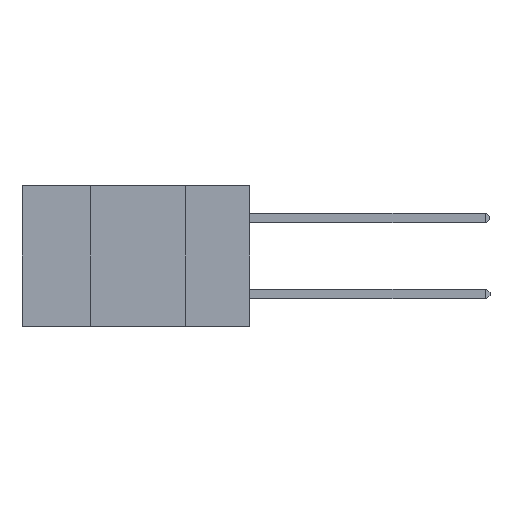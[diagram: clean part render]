
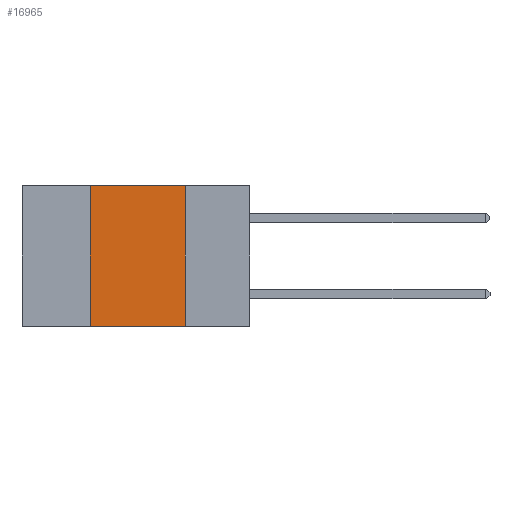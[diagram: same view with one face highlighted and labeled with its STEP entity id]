
A CAD part, left-side view. The second image highlights one B-rep face of the part: STEP entity #16965.
In plain terms, the highlighted planar face has unit normal (-1, 0, 0).
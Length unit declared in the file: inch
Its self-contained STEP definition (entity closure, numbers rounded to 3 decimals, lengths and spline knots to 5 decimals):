
#75 = VERTEX_POINT ( 'NONE', #18844 ) ;
#281 = VECTOR ( 'NONE', #6144, 39.37008 ) ;
#296 = ORIENTED_EDGE ( 'NONE', *, *, #1115, .T. ) ;
#842 = EDGE_CURVE ( 'NONE', #16833, #14727, #7809, .T. ) ;
#1115 = EDGE_CURVE ( 'NONE', #21065, #75, #10470, .T. ) ;
#2721 = VECTOR ( 'NONE', #24022, 39.37008 ) ;
#3122 = VECTOR ( 'NONE', #20569, 39.37008 ) ;
#3736 = PLANE ( 'NONE',  #4508 ) ;
#4141 = EDGE_LOOP ( 'NONE', ( #6253, #20050, #22191, #296 ) ) ;
#4332 = EDGE_CURVE ( 'NONE', #21065, #16833, #20109, .T. ) ;
#4508 = AXIS2_PLACEMENT_3D ( 'NONE', #24565, #17148, #13351 ) ;
#5139 = CARTESIAN_POINT ( 'NONE',  ( 0., 0.17, 0. ) ) ;
#5744 = FACE_OUTER_BOUND ( 'NONE', #4141, .T. ) ;
#6103 = VECTOR ( 'NONE', #9404, 39.37008 ) ;
#6144 = DIRECTION ( 'NONE',  ( 0., -1., 0. ) ) ;
#6253 = ORIENTED_EDGE ( 'NONE', *, *, #22015, .F. ) ;
#6368 = CARTESIAN_POINT ( 'NONE',  ( 0., 0.42, -0.37 ) ) ;
#7809 = LINE ( 'NONE', #12069, #2721 ) ;
#9404 = DIRECTION ( 'NONE',  ( 0., 0., -1. ) ) ;
#9707 = CARTESIAN_POINT ( 'NONE',  ( 0., 0.6, -0.37 ) ) ;
#10470 = LINE ( 'NONE', #9707, #281 ) ;
#11851 = LINE ( 'NONE', #17025, #6103 ) ;
#12069 = CARTESIAN_POINT ( 'NONE',  ( 0., 0.6, 0. ) ) ;
#13351 = DIRECTION ( 'NONE',  ( 0., 0., -1. ) ) ;
#14382 = CARTESIAN_POINT ( 'NONE',  ( 0., 0.42, 0. ) ) ;
#14727 = VERTEX_POINT ( 'NONE', #5139 ) ;
#16833 = VERTEX_POINT ( 'NONE', #14382 ) ;
#16965 = ADVANCED_FACE ( 'NONE', ( #5744 ), #3736, .F. ) ;
#17025 = CARTESIAN_POINT ( 'NONE',  ( 0., 0.17, 0. ) ) ;
#17148 = DIRECTION ( 'NONE',  ( 1., 0., 0. ) ) ;
#18674 = CARTESIAN_POINT ( 'NONE',  ( 0., 0.42, 0. ) ) ;
#18844 = CARTESIAN_POINT ( 'NONE',  ( 0., 0.17, -0.37 ) ) ;
#20050 = ORIENTED_EDGE ( 'NONE', *, *, #842, .F. ) ;
#20109 = LINE ( 'NONE', #18674, #3122 ) ;
#20569 = DIRECTION ( 'NONE',  ( 0., 0., 1. ) ) ;
#21065 = VERTEX_POINT ( 'NONE', #6368 ) ;
#22015 = EDGE_CURVE ( 'NONE', #14727, #75, #11851, .T. ) ;
#22191 = ORIENTED_EDGE ( 'NONE', *, *, #4332, .F. ) ;
#24022 = DIRECTION ( 'NONE',  ( 0., -1., 0. ) ) ;
#24565 = CARTESIAN_POINT ( 'NONE',  ( 0., 0.6, 0. ) ) ;
